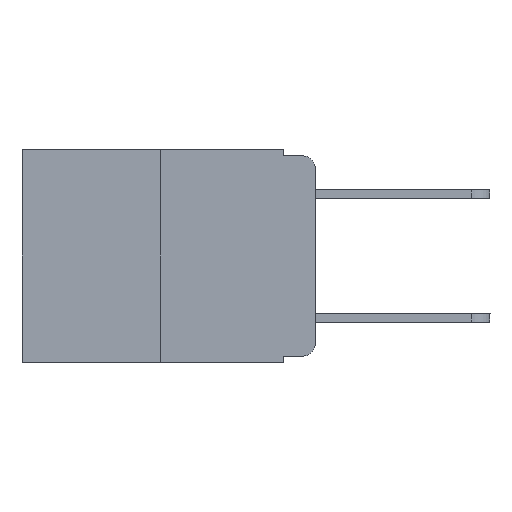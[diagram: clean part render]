
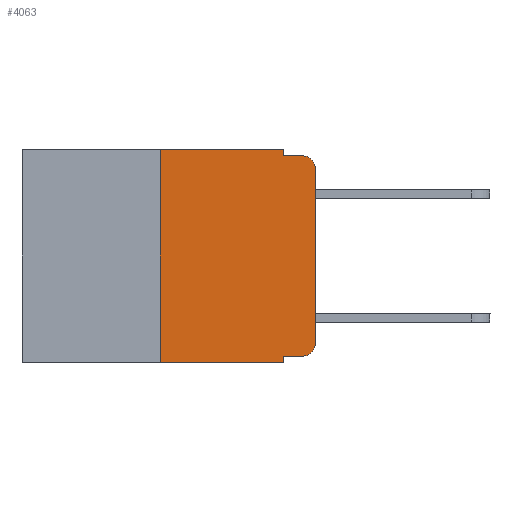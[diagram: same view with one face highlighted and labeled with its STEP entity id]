
A CAD part, left-side view. The second image highlights one B-rep face of the part: STEP entity #4063.
In plain terms, the highlighted planar face has unit normal (-1, 0, 0).
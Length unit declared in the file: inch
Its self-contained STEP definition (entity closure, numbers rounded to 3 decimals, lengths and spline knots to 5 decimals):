
#45 = DIRECTION ( 'NONE',  ( 0., 0., 1. ) ) ;
#249 = CARTESIAN_POINT ( 'NONE',  ( 0., 0.473, -0.343 ) ) ;
#810 = CARTESIAN_POINT ( 'NONE',  ( 0., 0.25, 0. ) ) ;
#895 = ORIENTED_EDGE ( 'NONE', *, *, #9766, .F. ) ;
#917 = EDGE_CURVE ( 'NONE', #2205, #9084, #3299, .T. ) ;
#1048 = ORIENTED_EDGE ( 'NONE', *, *, #8683, .T. ) ;
#1070 = DIRECTION ( 'NONE',  ( 0., 0., -1. ) ) ;
#1217 = DIRECTION ( 'NONE',  ( 0., -1., 0. ) ) ;
#1268 = VECTOR ( 'NONE', #1217, 39.37008 ) ;
#1430 = VERTEX_POINT ( 'NONE', #5994 ) ;
#1567 = EDGE_CURVE ( 'NONE', #6612, #3400, #4177, .T. ) ;
#1724 = DIRECTION ( 'NONE',  ( 0., -1., 0. ) ) ;
#1731 = CARTESIAN_POINT ( 'NONE',  ( 0., 0., -0.313 ) ) ;
#1836 = VERTEX_POINT ( 'NONE', #2952 ) ;
#1895 = ORIENTED_EDGE ( 'NONE', *, *, #4519, .F. ) ;
#1902 = AXIS2_PLACEMENT_3D ( 'NONE', #5973, #2059, #7704 ) ;
#1910 = PLANE ( 'NONE',  #2542 ) ;
#2059 = DIRECTION ( 'NONE',  ( -1., 0., 0. ) ) ;
#2070 = ORIENTED_EDGE ( 'NONE', *, *, #5756, .T. ) ;
#2095 = VECTOR ( 'NONE', #8060, 39.37008 ) ;
#2166 = ORIENTED_EDGE ( 'NONE', *, *, #917, .F. ) ;
#2167 = CARTESIAN_POINT ( 'NONE',  ( 0., 0., 0. ) ) ;
#2205 = VERTEX_POINT ( 'NONE', #9200 ) ;
#2339 = VECTOR ( 'NONE', #1724, 39.37008 ) ;
#2542 = AXIS2_PLACEMENT_3D ( 'NONE', #8500, #8439, #10100 ) ;
#2636 = CARTESIAN_POINT ( 'NONE',  ( 0., 0., -0.03 ) ) ;
#2952 = CARTESIAN_POINT ( 'NONE',  ( 0., 0.25, 0. ) ) ;
#3008 = CIRCLE ( 'NONE', #8504, 0.02 ) ;
#3032 = CARTESIAN_POINT ( 'NONE',  ( 0., 0.051, -0.01 ) ) ;
#3038 = VECTOR ( 'NONE', #7788, 39.37008 ) ;
#3224 = LINE ( 'NONE', #6618, #2339 ) ;
#3227 = CARTESIAN_POINT ( 'NONE',  ( 0., 0.051, -0.343 ) ) ;
#3299 = LINE ( 'NONE', #5396, #3038 ) ;
#3400 = VERTEX_POINT ( 'NONE', #3032 ) ;
#3494 = DIRECTION ( 'NONE',  ( -1., 0., 0. ) ) ;
#3697 = VERTEX_POINT ( 'NONE', #2636 ) ;
#3725 = EDGE_CURVE ( 'NONE', #5563, #9084, #5525, .T. ) ;
#3760 = EDGE_CURVE ( 'NONE', #3400, #1430, #6807, .T. ) ;
#3803 = DIRECTION ( 'NONE',  ( 0., 0., 1. ) ) ;
#4045 = DIRECTION ( 'NONE',  ( 0., -1., 0. ) ) ;
#4063 = ADVANCED_FACE ( 'NONE', ( #10324 ), #1910, .F. ) ;
#4177 = LINE ( 'NONE', #4260, #5451 ) ;
#4211 = ORIENTED_EDGE ( 'NONE', *, *, #3725, .T. ) ;
#4222 = VECTOR ( 'NONE', #3803, 39.37008 ) ;
#4260 = CARTESIAN_POINT ( 'NONE',  ( 0., 0.051, 0. ) ) ;
#4365 = CARTESIAN_POINT ( 'NONE',  ( 0., 0.051, -0.333 ) ) ;
#4519 = EDGE_CURVE ( 'NONE', #5563, #1836, #9183, .T. ) ;
#4771 = EDGE_LOOP ( 'NONE', ( #9030, #6726, #10212, #5001, #895, #1895, #4211, #2166, #2070, #1048 ) ) ;
#5001 = ORIENTED_EDGE ( 'NONE', *, *, #1567, .F. ) ;
#5013 = DIRECTION ( 'NONE',  ( 0., 0., -1. ) ) ;
#5369 = LINE ( 'NONE', #2167, #4222 ) ;
#5396 = CARTESIAN_POINT ( 'NONE',  ( 0., 0.051, 0. ) ) ;
#5451 = VECTOR ( 'NONE', #1070, 39.37008 ) ;
#5525 = LINE ( 'NONE', #249, #2095 ) ;
#5563 = VERTEX_POINT ( 'NONE', #5598 ) ;
#5598 = CARTESIAN_POINT ( 'NONE',  ( 0., 0.25, -0.343 ) ) ;
#5756 = EDGE_CURVE ( 'NONE', #2205, #10111, #7375, .T. ) ;
#5973 = CARTESIAN_POINT ( 'NONE',  ( 0., 0.02, -0.313 ) ) ;
#5994 = CARTESIAN_POINT ( 'NONE',  ( 0., 0.02, -0.01 ) ) ;
#6072 = CARTESIAN_POINT ( 'NONE',  ( 0., 0.02, -0.333 ) ) ;
#6176 = VERTEX_POINT ( 'NONE', #1731 ) ;
#6276 = EDGE_CURVE ( 'NONE', #3697, #1430, #3008, .T. ) ;
#6612 = VERTEX_POINT ( 'NONE', #7009 ) ;
#6618 = CARTESIAN_POINT ( 'NONE',  ( 0., 0.473, 0. ) ) ;
#6726 = ORIENTED_EDGE ( 'NONE', *, *, #6276, .T. ) ;
#6807 = LINE ( 'NONE', #7291, #10253 ) ;
#7009 = CARTESIAN_POINT ( 'NONE',  ( 0., 0.051, 0. ) ) ;
#7291 = CARTESIAN_POINT ( 'NONE',  ( 0., 0.051, -0.01 ) ) ;
#7375 = LINE ( 'NONE', #4365, #1268 ) ;
#7704 = DIRECTION ( 'NONE',  ( 0., 0., -1. ) ) ;
#7788 = DIRECTION ( 'NONE',  ( 0., 0., -1. ) ) ;
#8060 = DIRECTION ( 'NONE',  ( 0., -1., 0. ) ) ;
#8439 = DIRECTION ( 'NONE',  ( 1., 0., 0. ) ) ;
#8500 = CARTESIAN_POINT ( 'NONE',  ( 0., 0.473, 0. ) ) ;
#8504 = AXIS2_PLACEMENT_3D ( 'NONE', #9879, #3494, #5013 ) ;
#8683 = EDGE_CURVE ( 'NONE', #10111, #6176, #9267, .T. ) ;
#9030 = ORIENTED_EDGE ( 'NONE', *, *, #10151, .T. ) ;
#9046 = VECTOR ( 'NONE', #45, 39.37008 ) ;
#9084 = VERTEX_POINT ( 'NONE', #3227 ) ;
#9183 = LINE ( 'NONE', #810, #9046 ) ;
#9200 = CARTESIAN_POINT ( 'NONE',  ( 0., 0.051, -0.333 ) ) ;
#9267 = CIRCLE ( 'NONE', #1902, 0.02 ) ;
#9766 = EDGE_CURVE ( 'NONE', #1836, #6612, #3224, .T. ) ;
#9879 = CARTESIAN_POINT ( 'NONE',  ( 0., 0.02, -0.03 ) ) ;
#10100 = DIRECTION ( 'NONE',  ( 0., 0., -1. ) ) ;
#10111 = VERTEX_POINT ( 'NONE', #6072 ) ;
#10151 = EDGE_CURVE ( 'NONE', #6176, #3697, #5369, .T. ) ;
#10212 = ORIENTED_EDGE ( 'NONE', *, *, #3760, .F. ) ;
#10253 = VECTOR ( 'NONE', #4045, 39.37008 ) ;
#10324 = FACE_OUTER_BOUND ( 'NONE', #4771, .T. ) ;
